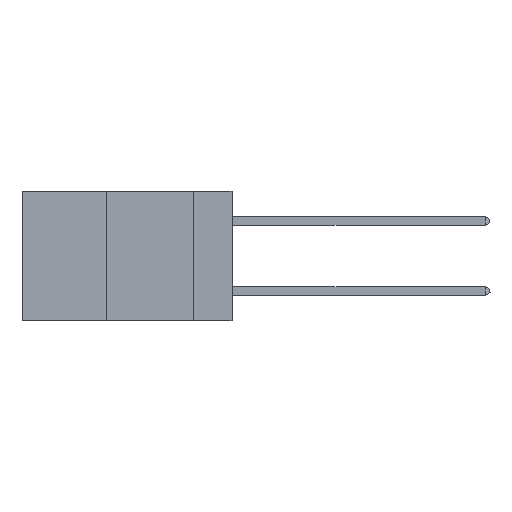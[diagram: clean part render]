
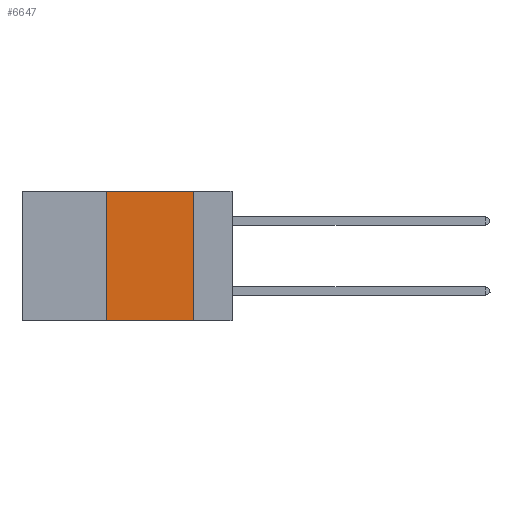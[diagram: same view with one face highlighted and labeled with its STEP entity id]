
A CAD part, left-side view. The second image highlights one B-rep face of the part: STEP entity #6647.
In plain terms, the highlighted planar face has unit normal (-1, 0, 0).
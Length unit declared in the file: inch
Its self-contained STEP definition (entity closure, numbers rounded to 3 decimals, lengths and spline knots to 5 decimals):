
#55 = LINE ( 'NONE', #6940, #1803 ) ;
#775 = CARTESIAN_POINT ( 'NONE',  ( 0., 0.11, -0.37 ) ) ;
#1803 = VECTOR ( 'NONE', #28495, 39.37008 ) ;
#4104 = DIRECTION ( 'NONE',  ( 0., -1., 0. ) ) ;
#5626 = EDGE_CURVE ( 'NONE', #8657, #20236, #26749, .T. ) ;
#6647 = ADVANCED_FACE ( 'NONE', ( #9968 ), #32693, .F. ) ;
#6940 = CARTESIAN_POINT ( 'NONE',  ( 0., 0.11, 0. ) ) ;
#7647 = ORIENTED_EDGE ( 'NONE', *, *, #32237, .F. ) ;
#7745 = DIRECTION ( 'NONE',  ( 0., 0., 1. ) ) ;
#8280 = VECTOR ( 'NONE', #7745, 39.37008 ) ;
#8657 = VERTEX_POINT ( 'NONE', #34144 ) ;
#9968 = FACE_OUTER_BOUND ( 'NONE', #29978, .T. ) ;
#10108 = EDGE_CURVE ( 'NONE', #15285, #26712, #15725, .T. ) ;
#11277 = DIRECTION ( 'NONE',  ( 0., 0., -1. ) ) ;
#12251 = ORIENTED_EDGE ( 'NONE', *, *, #10108, .T. ) ;
#15285 = VERTEX_POINT ( 'NONE', #32466 ) ;
#15725 = LINE ( 'NONE', #27298, #31149 ) ;
#17407 = AXIS2_PLACEMENT_3D ( 'NONE', #22156, #19179, #11277 ) ;
#19179 = DIRECTION ( 'NONE',  ( 1., 0., 0. ) ) ;
#20236 = VERTEX_POINT ( 'NONE', #25110 ) ;
#20949 = ORIENTED_EDGE ( 'NONE', *, *, #5626, .F. ) ;
#22156 = CARTESIAN_POINT ( 'NONE',  ( 0., 0.6, 0. ) ) ;
#23236 = CARTESIAN_POINT ( 'NONE',  ( 0., 0.6, 0. ) ) ;
#23285 = LINE ( 'NONE', #30975, #8280 ) ;
#25110 = CARTESIAN_POINT ( 'NONE',  ( 0., 0.11, 0. ) ) ;
#25729 = DIRECTION ( 'NONE',  ( 0., -1., 0. ) ) ;
#26712 = VERTEX_POINT ( 'NONE', #775 ) ;
#26749 = LINE ( 'NONE', #23236, #31887 ) ;
#27298 = CARTESIAN_POINT ( 'NONE',  ( 0., 0.6, -0.37 ) ) ;
#28495 = DIRECTION ( 'NONE',  ( 0., 0., -1. ) ) ;
#29978 = EDGE_LOOP ( 'NONE', ( #7647, #20949, #33702, #12251 ) ) ;
#30975 = CARTESIAN_POINT ( 'NONE',  ( 0., 0.36, 0. ) ) ;
#31149 = VECTOR ( 'NONE', #4104, 39.37008 ) ;
#31887 = VECTOR ( 'NONE', #25729, 39.37008 ) ;
#32148 = EDGE_CURVE ( 'NONE', #15285, #8657, #23285, .T. ) ;
#32237 = EDGE_CURVE ( 'NONE', #20236, #26712, #55, .T. ) ;
#32466 = CARTESIAN_POINT ( 'NONE',  ( 0., 0.36, -0.37 ) ) ;
#32693 = PLANE ( 'NONE',  #17407 ) ;
#33702 = ORIENTED_EDGE ( 'NONE', *, *, #32148, .F. ) ;
#34144 = CARTESIAN_POINT ( 'NONE',  ( 0., 0.36, 0. ) ) ;
